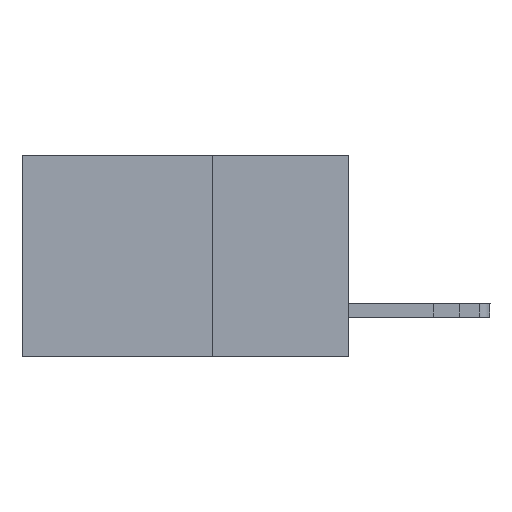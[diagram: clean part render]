
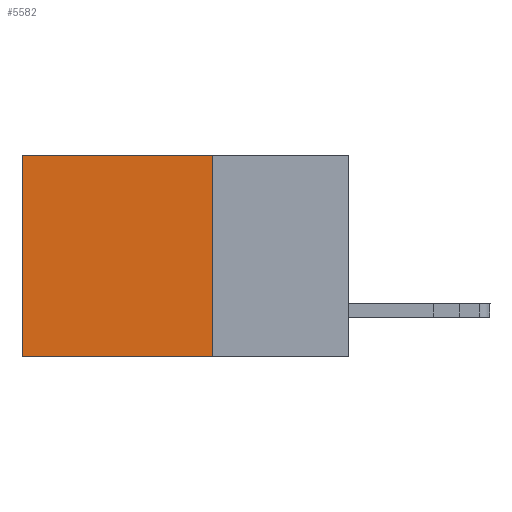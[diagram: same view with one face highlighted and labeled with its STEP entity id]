
A CAD part, left-side view. The second image highlights one B-rep face of the part: STEP entity #5582.
In plain terms, the highlighted planar face has unit normal (-1, 0, 0).
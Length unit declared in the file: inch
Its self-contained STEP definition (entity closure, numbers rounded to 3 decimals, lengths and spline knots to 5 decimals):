
#376 = VECTOR ( 'NONE', #13976, 39.37008 ) ;
#879 = VERTEX_POINT ( 'NONE', #6835 ) ;
#1896 = LINE ( 'NONE', #4534, #8546 ) ;
#2294 = EDGE_CURVE ( 'NONE', #10631, #879, #4992, .T. ) ;
#2965 = CARTESIAN_POINT ( 'NONE',  ( 0.298, 0.6, 0. ) ) ;
#3124 = DIRECTION ( 'NONE',  ( 0., 1., 0. ) ) ;
#3717 = EDGE_CURVE ( 'NONE', #10815, #5741, #1896, .T. ) ;
#4144 = ORIENTED_EDGE ( 'NONE', *, *, #3717, .T. ) ;
#4430 = DIRECTION ( 'NONE',  ( 0., 0., -1. ) ) ;
#4534 = CARTESIAN_POINT ( 'NONE',  ( 0.298, 0.25, 0. ) ) ;
#4992 = LINE ( 'NONE', #14538, #15312 ) ;
#5037 = PLANE ( 'NONE',  #8869 ) ;
#5341 = EDGE_CURVE ( 'NONE', #5741, #879, #13346, .T. ) ;
#5582 = ADVANCED_FACE ( 'NONE', ( #12563 ), #5037, .F. ) ;
#5741 = VERTEX_POINT ( 'NONE', #2965 ) ;
#6201 = VECTOR ( 'NONE', #4430, 39.37008 ) ;
#6398 = CARTESIAN_POINT ( 'NONE',  ( 0.298, 0.25, -0.37 ) ) ;
#6656 = EDGE_LOOP ( 'NONE', ( #11237, #10671, #12582, #4144 ) ) ;
#6835 = CARTESIAN_POINT ( 'NONE',  ( 0.298, 0.6, -0.37 ) ) ;
#7056 = EDGE_CURVE ( 'NONE', #10815, #10631, #8256, .T. ) ;
#7182 = DIRECTION ( 'NONE',  ( 0., 1., 0. ) ) ;
#8256 = LINE ( 'NONE', #12988, #6201 ) ;
#8546 = VECTOR ( 'NONE', #3124, 39.37008 ) ;
#8690 = CARTESIAN_POINT ( 'NONE',  ( 0.298, 0.25, 0. ) ) ;
#8869 = AXIS2_PLACEMENT_3D ( 'NONE', #14833, #11075, #11020 ) ;
#10631 = VERTEX_POINT ( 'NONE', #6398 ) ;
#10671 = ORIENTED_EDGE ( 'NONE', *, *, #2294, .F. ) ;
#10815 = VERTEX_POINT ( 'NONE', #8690 ) ;
#11020 = DIRECTION ( 'NONE',  ( 0., 0., -1. ) ) ;
#11075 = DIRECTION ( 'NONE',  ( 1., 0., 0. ) ) ;
#11237 = ORIENTED_EDGE ( 'NONE', *, *, #5341, .T. ) ;
#11660 = CARTESIAN_POINT ( 'NONE',  ( 0.298, 0.6, 0. ) ) ;
#12563 = FACE_OUTER_BOUND ( 'NONE', #6656, .T. ) ;
#12582 = ORIENTED_EDGE ( 'NONE', *, *, #7056, .F. ) ;
#12988 = CARTESIAN_POINT ( 'NONE',  ( 0.298, 0.25, 0. ) ) ;
#13346 = LINE ( 'NONE', #11660, #376 ) ;
#13976 = DIRECTION ( 'NONE',  ( 0., 0., -1. ) ) ;
#14538 = CARTESIAN_POINT ( 'NONE',  ( 0.298, 0.25, -0.37 ) ) ;
#14833 = CARTESIAN_POINT ( 'NONE',  ( 0.298, 0.25, 0. ) ) ;
#15312 = VECTOR ( 'NONE', #7182, 39.37008 ) ;
